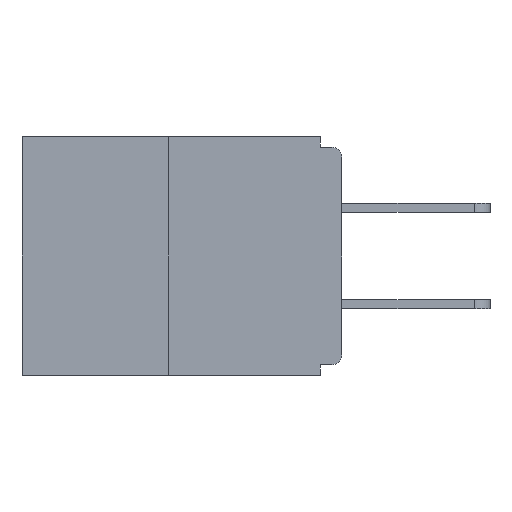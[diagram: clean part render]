
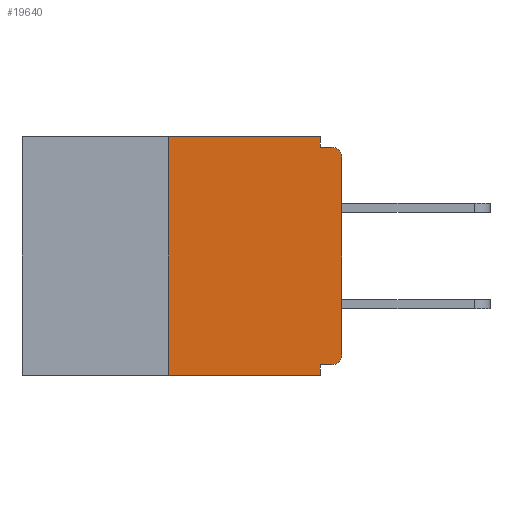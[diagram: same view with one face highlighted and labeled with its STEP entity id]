
A CAD part, left-side view. The second image highlights one B-rep face of the part: STEP entity #19640.
In plain terms, the highlighted planar face has unit normal (-1, 0, 0).
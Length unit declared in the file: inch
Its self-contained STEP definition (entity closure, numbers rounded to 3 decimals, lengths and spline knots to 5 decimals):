
#319 = DIRECTION ( 'NONE',  ( 0., 0., -1. ) ) ;
#692 = DIRECTION ( 'NONE',  ( -1., 0., 0. ) ) ;
#693 = CARTESIAN_POINT ( 'NONE',  ( 0., 0.031, -0.328 ) ) ;
#860 = DIRECTION ( 'NONE',  ( 0., 0., -1. ) ) ;
#895 = VERTEX_POINT ( 'NONE', #11851 ) ;
#1243 = CARTESIAN_POINT ( 'NONE',  ( 0., 0.25, 0. ) ) ;
#1525 = VECTOR ( 'NONE', #1708, 39.37008 ) ;
#1559 = VECTOR ( 'NONE', #17805, 39.37008 ) ;
#1676 = LINE ( 'NONE', #7712, #7374 ) ;
#1708 = DIRECTION ( 'NONE',  ( 0., 0., 1. ) ) ;
#1882 = VECTOR ( 'NONE', #860, 39.37008 ) ;
#2019 = VECTOR ( 'NONE', #18225, 39.37008 ) ;
#2240 = ORIENTED_EDGE ( 'NONE', *, *, #4417, .T. ) ;
#2249 = ORIENTED_EDGE ( 'NONE', *, *, #6582, .T. ) ;
#2506 = ORIENTED_EDGE ( 'NONE', *, *, #15707, .T. ) ;
#2714 = LINE ( 'NONE', #1243, #6460 ) ;
#2725 = CARTESIAN_POINT ( 'NONE',  ( 0., 0.25, -0.343 ) ) ;
#2806 = EDGE_CURVE ( 'NONE', #12187, #21222, #2714, .T. ) ;
#3341 = EDGE_CURVE ( 'NONE', #15236, #6456, #19999, .T. ) ;
#3976 = LINE ( 'NONE', #6114, #9620 ) ;
#4153 = PLANE ( 'NONE',  #16852 ) ;
#4417 = EDGE_CURVE ( 'NONE', #10840, #17900, #13156, .T. ) ;
#5684 = CARTESIAN_POINT ( 'NONE',  ( 0., 0., -0.03 ) ) ;
#5900 = ORIENTED_EDGE ( 'NONE', *, *, #3341, .T. ) ;
#6114 = CARTESIAN_POINT ( 'NONE',  ( 0., 0., -0.015 ) ) ;
#6279 = VERTEX_POINT ( 'NONE', #693 ) ;
#6456 = VERTEX_POINT ( 'NONE', #8524 ) ;
#6460 = VECTOR ( 'NONE', #22070, 39.37008 ) ;
#6582 = EDGE_CURVE ( 'NONE', #6456, #10840, #12322, .T. ) ;
#7374 = VECTOR ( 'NONE', #13080, 39.37008 ) ;
#7712 = CARTESIAN_POINT ( 'NONE',  ( 0., 0.031, 0. ) ) ;
#7793 = CARTESIAN_POINT ( 'NONE',  ( 0., 0.46, 0. ) ) ;
#8009 = EDGE_CURVE ( 'NONE', #15236, #6279, #19905, .T. ) ;
#8146 = CARTESIAN_POINT ( 'NONE',  ( 0., 0.015, -0.015 ) ) ;
#8524 = CARTESIAN_POINT ( 'NONE',  ( 0., 0., -0.313 ) ) ;
#8736 = VERTEX_POINT ( 'NONE', #19297 ) ;
#9572 = DIRECTION ( 'NONE',  ( 1., 0., 0. ) ) ;
#9620 = VECTOR ( 'NONE', #13123, 39.37008 ) ;
#9889 = CARTESIAN_POINT ( 'NONE',  ( 0., 0.031, -0.343 ) ) ;
#10449 = CARTESIAN_POINT ( 'NONE',  ( 0., 0.46, -0.343 ) ) ;
#10520 = DIRECTION ( 'NONE',  ( 0., 0., -1. ) ) ;
#10760 = FACE_OUTER_BOUND ( 'NONE', #17461, .T. ) ;
#10840 = VERTEX_POINT ( 'NONE', #5684 ) ;
#10906 = CARTESIAN_POINT ( 'NONE',  ( 0., 0., 0. ) ) ;
#11379 = CARTESIAN_POINT ( 'NONE',  ( 0., 0.015, -0.328 ) ) ;
#11851 = CARTESIAN_POINT ( 'NONE',  ( 0., 0.031, -0.015 ) ) ;
#12107 = DIRECTION ( 'NONE',  ( -1., 0., 0. ) ) ;
#12187 = VERTEX_POINT ( 'NONE', #2725 ) ;
#12322 = LINE ( 'NONE', #10906, #1525 ) ;
#12368 = LINE ( 'NONE', #9889, #1882 ) ;
#12875 = ORIENTED_EDGE ( 'NONE', *, *, #19041, .F. ) ;
#13080 = DIRECTION ( 'NONE',  ( 0., 0., -1. ) ) ;
#13123 = DIRECTION ( 'NONE',  ( 0., -1., 0. ) ) ;
#13156 = CIRCLE ( 'NONE', #21615, 0.015 ) ;
#13226 = EDGE_CURVE ( 'NONE', #895, #17900, #3976, .T. ) ;
#13296 = DIRECTION ( 'NONE',  ( 0., 0., -1. ) ) ;
#14508 = AXIS2_PLACEMENT_3D ( 'NONE', #22940, #12107, #10520 ) ;
#14639 = LINE ( 'NONE', #10449, #1559 ) ;
#14852 = VECTOR ( 'NONE', #19413, 39.37008 ) ;
#15236 = VERTEX_POINT ( 'NONE', #11379 ) ;
#15367 = ORIENTED_EDGE ( 'NONE', *, *, #8009, .F. ) ;
#15436 = CARTESIAN_POINT ( 'NONE',  ( 0., 0.031, -0.343 ) ) ;
#15707 = EDGE_CURVE ( 'NONE', #12187, #17864, #14639, .T. ) ;
#15894 = LINE ( 'NONE', #21614, #2019 ) ;
#15943 = ORIENTED_EDGE ( 'NONE', *, *, #13226, .F. ) ;
#16260 = CARTESIAN_POINT ( 'NONE',  ( 0., 0.25, 0. ) ) ;
#16852 = AXIS2_PLACEMENT_3D ( 'NONE', #7793, #9572, #319 ) ;
#17055 = ORIENTED_EDGE ( 'NONE', *, *, #22367, .F. ) ;
#17461 = EDGE_LOOP ( 'NONE', ( #12875, #20885, #2506, #17055, #15367, #5900, #2249, #2240, #15943, #23315 ) ) ;
#17598 = CARTESIAN_POINT ( 'NONE',  ( 0., 0., -0.328 ) ) ;
#17805 = DIRECTION ( 'NONE',  ( 0., -1., 0. ) ) ;
#17864 = VERTEX_POINT ( 'NONE', #15436 ) ;
#17900 = VERTEX_POINT ( 'NONE', #8146 ) ;
#18225 = DIRECTION ( 'NONE',  ( 0., -1., 0. ) ) ;
#19041 = EDGE_CURVE ( 'NONE', #21222, #8736, #15894, .T. ) ;
#19297 = CARTESIAN_POINT ( 'NONE',  ( 0., 0.031, 0. ) ) ;
#19413 = DIRECTION ( 'NONE',  ( 0., 1., 0. ) ) ;
#19617 = EDGE_CURVE ( 'NONE', #8736, #895, #1676, .T. ) ;
#19640 = ADVANCED_FACE ( 'NONE', ( #10760 ), #4153, .F. ) ;
#19905 = LINE ( 'NONE', #17598, #14852 ) ;
#19999 = CIRCLE ( 'NONE', #14508, 0.015 ) ;
#20086 = CARTESIAN_POINT ( 'NONE',  ( 0., 0.015, -0.03 ) ) ;
#20885 = ORIENTED_EDGE ( 'NONE', *, *, #2806, .F. ) ;
#21222 = VERTEX_POINT ( 'NONE', #16260 ) ;
#21615 = AXIS2_PLACEMENT_3D ( 'NONE', #20086, #692, #13296 ) ;
#21614 = CARTESIAN_POINT ( 'NONE',  ( 0., 0.46, 0. ) ) ;
#22070 = DIRECTION ( 'NONE',  ( 0., 0., 1. ) ) ;
#22367 = EDGE_CURVE ( 'NONE', #6279, #17864, #12368, .T. ) ;
#22940 = CARTESIAN_POINT ( 'NONE',  ( 0., 0.015, -0.313 ) ) ;
#23315 = ORIENTED_EDGE ( 'NONE', *, *, #19617, .F. ) ;
